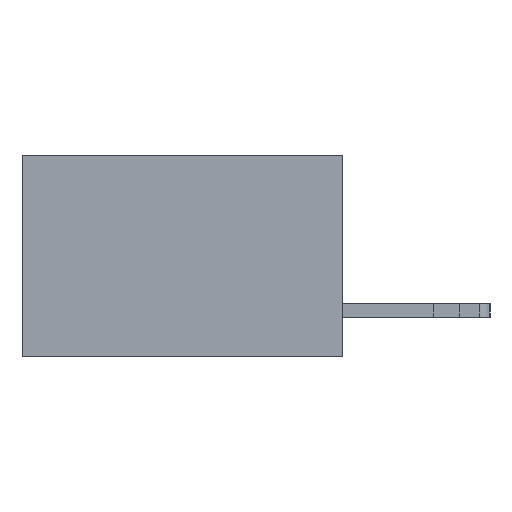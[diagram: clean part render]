
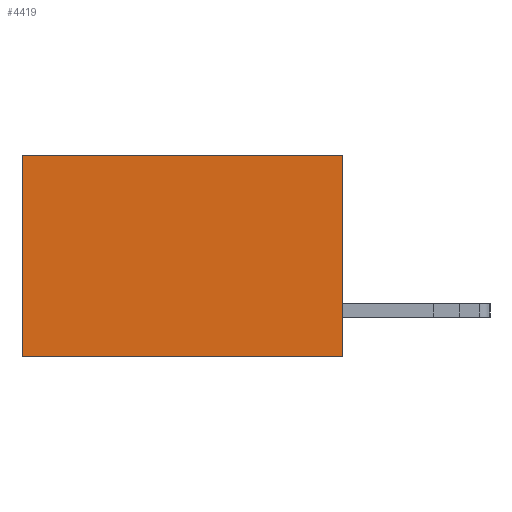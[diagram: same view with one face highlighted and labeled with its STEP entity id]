
A CAD part, left-side view. The second image highlights one B-rep face of the part: STEP entity #4419.
In plain terms, the highlighted planar face has unit normal (-1, 0, 0).
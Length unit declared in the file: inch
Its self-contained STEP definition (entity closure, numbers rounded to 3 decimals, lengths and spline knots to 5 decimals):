
#60 = CARTESIAN_POINT ( 'NONE',  ( 0.277, 0., -0.37 ) ) ;
#1492 = VERTEX_POINT ( 'NONE', #10748 ) ;
#1706 = DIRECTION ( 'NONE',  ( 0., 1., 0. ) ) ;
#1771 = LINE ( 'NONE', #5850, #16399 ) ;
#2044 = LINE ( 'NONE', #7046, #8737 ) ;
#2977 = EDGE_CURVE ( 'NONE', #3170, #1492, #17735, .T. ) ;
#3170 = VERTEX_POINT ( 'NONE', #16889 ) ;
#3656 = VERTEX_POINT ( 'NONE', #8287 ) ;
#3798 = VERTEX_POINT ( 'NONE', #12919 ) ;
#4419 = ADVANCED_FACE ( 'NONE', ( #12709 ), #6277, .F. ) ;
#5850 = CARTESIAN_POINT ( 'NONE',  ( 0.277, 0., -0.37 ) ) ;
#6219 = DIRECTION ( 'NONE',  ( 0., 0., -1. ) ) ;
#6237 = DIRECTION ( 'NONE',  ( 1., 0., 0. ) ) ;
#6277 = PLANE ( 'NONE',  #8792 ) ;
#6311 = CARTESIAN_POINT ( 'NONE',  ( 0.277, 0., -0.37 ) ) ;
#7046 = CARTESIAN_POINT ( 'NONE',  ( 0.277, 0.59, -0.37 ) ) ;
#8287 = CARTESIAN_POINT ( 'NONE',  ( 0.277, 0.59, -0.37 ) ) ;
#8434 = ORIENTED_EDGE ( 'NONE', *, *, #2977, .T. ) ;
#8737 = VECTOR ( 'NONE', #14108, 39.37008 ) ;
#8792 = AXIS2_PLACEMENT_3D ( 'NONE', #6311, #6237, #6219 ) ;
#8924 = EDGE_CURVE ( 'NONE', #1492, #3656, #2044, .T. ) ;
#9134 = CARTESIAN_POINT ( 'NONE',  ( 0.277, 0., 0. ) ) ;
#9508 = DIRECTION ( 'NONE',  ( 0., 1., 0. ) ) ;
#9870 = VECTOR ( 'NONE', #1706, 39.37008 ) ;
#10642 = EDGE_CURVE ( 'NONE', #3170, #3798, #1771, .T. ) ;
#10748 = CARTESIAN_POINT ( 'NONE',  ( 0.277, 0.59, 0. ) ) ;
#12709 = FACE_OUTER_BOUND ( 'NONE', #16573, .T. ) ;
#12919 = CARTESIAN_POINT ( 'NONE',  ( 0.277, 0., -0.37 ) ) ;
#13471 = EDGE_CURVE ( 'NONE', #3798, #3656, #17723, .T. ) ;
#14108 = DIRECTION ( 'NONE',  ( 0., 0., -1. ) ) ;
#14238 = ORIENTED_EDGE ( 'NONE', *, *, #13471, .F. ) ;
#16399 = VECTOR ( 'NONE', #17108, 39.37008 ) ;
#16573 = EDGE_LOOP ( 'NONE', ( #16616, #14238, #18140, #8434 ) ) ;
#16616 = ORIENTED_EDGE ( 'NONE', *, *, #8924, .T. ) ;
#16889 = CARTESIAN_POINT ( 'NONE',  ( 0.277, 0., 0. ) ) ;
#17108 = DIRECTION ( 'NONE',  ( 0., 0., -1. ) ) ;
#17311 = VECTOR ( 'NONE', #9508, 39.37008 ) ;
#17723 = LINE ( 'NONE', #60, #9870 ) ;
#17735 = LINE ( 'NONE', #9134, #17311 ) ;
#18140 = ORIENTED_EDGE ( 'NONE', *, *, #10642, .F. ) ;
